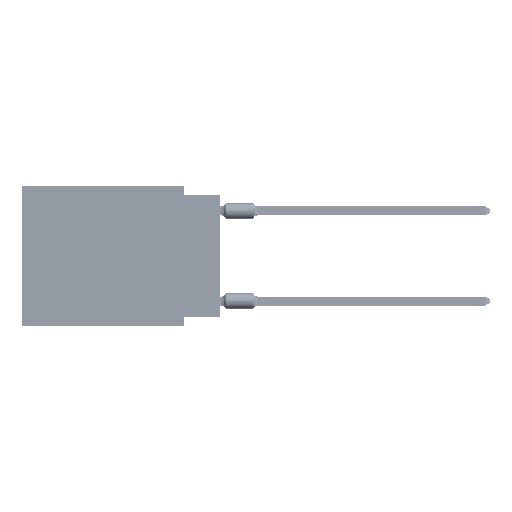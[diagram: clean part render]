
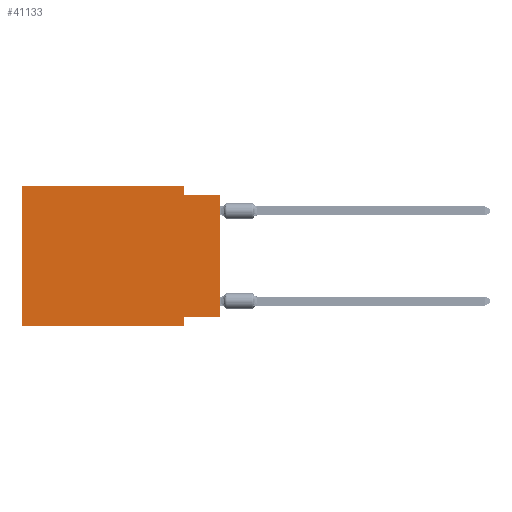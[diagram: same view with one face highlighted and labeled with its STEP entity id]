
A CAD part, left-side view. The second image highlights one B-rep face of the part: STEP entity #41133.
In plain terms, the highlighted planar face has unit normal (-1, 0, 0).
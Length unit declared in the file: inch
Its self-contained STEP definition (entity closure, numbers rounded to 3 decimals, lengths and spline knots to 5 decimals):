
#1566 = CARTESIAN_POINT ( 'NONE',  ( 0., 0., -0.025 ) ) ;
#3106 = LINE ( 'NONE', #46605, #52189 ) ;
#8135 = LINE ( 'NONE', #40934, #17220 ) ;
#8172 = EDGE_CURVE ( 'NONE', #58914, #65936, #8135, .T. ) ;
#9421 = VECTOR ( 'NONE', #50061, 39.37008 ) ;
#10401 = CARTESIAN_POINT ( 'NONE',  ( 0., 0.55, -0.39 ) ) ;
#13799 = DIRECTION ( 'NONE',  ( 0., 0., 1. ) ) ;
#14535 = CARTESIAN_POINT ( 'NONE',  ( 0., 0., -0.365 ) ) ;
#14879 = EDGE_CURVE ( 'NONE', #18918, #38628, #37913, .T. ) ;
#16019 = EDGE_CURVE ( 'NONE', #68452, #18918, #46239, .T. ) ;
#16567 = LINE ( 'NONE', #22951, #9421 ) ;
#16810 = VECTOR ( 'NONE', #13799, 39.37008 ) ;
#16828 = LINE ( 'NONE', #10401, #68112 ) ;
#17159 = DIRECTION ( 'NONE',  ( 0., -1., 0. ) ) ;
#17220 = VECTOR ( 'NONE', #62311, 39.37008 ) ;
#18135 = DIRECTION ( 'NONE',  ( 0., 0., -1. ) ) ;
#18264 = ORIENTED_EDGE ( 'NONE', *, *, #30459, .T. ) ;
#18918 = VERTEX_POINT ( 'NONE', #27631 ) ;
#18987 = FACE_OUTER_BOUND ( 'NONE', #70280, .T. ) ;
#21227 = VECTOR ( 'NONE', #37195, 39.37008 ) ;
#22951 = CARTESIAN_POINT ( 'NONE',  ( 0., 0., -0.025 ) ) ;
#23800 = ORIENTED_EDGE ( 'NONE', *, *, #62134, .T. ) ;
#23830 = LINE ( 'NONE', #61618, #54489 ) ;
#24163 = ORIENTED_EDGE ( 'NONE', *, *, #16019, .F. ) ;
#26587 = EDGE_CURVE ( 'NONE', #38628, #33888, #23830, .T. ) ;
#27631 = CARTESIAN_POINT ( 'NONE',  ( 0., 0.55, 0. ) ) ;
#29457 = CARTESIAN_POINT ( 'NONE',  ( 0., 0.1, 0. ) ) ;
#30459 = EDGE_CURVE ( 'NONE', #58914, #63016, #69448, .T. ) ;
#33888 = VERTEX_POINT ( 'NONE', #38398 ) ;
#35043 = CARTESIAN_POINT ( 'NONE',  ( 0., 0.55, 0. ) ) ;
#35385 = DIRECTION ( 'NONE',  ( 0., 0., -1. ) ) ;
#37195 = DIRECTION ( 'NONE',  ( 0., -1., 0. ) ) ;
#37747 = CARTESIAN_POINT ( 'NONE',  ( 0., 0., 0. ) ) ;
#37913 = LINE ( 'NONE', #64629, #21227 ) ;
#38398 = CARTESIAN_POINT ( 'NONE',  ( 0., 0.1, -0.025 ) ) ;
#38628 = VERTEX_POINT ( 'NONE', #29457 ) ;
#40934 = CARTESIAN_POINT ( 'NONE',  ( 0., 0., -0.365 ) ) ;
#41133 = ADVANCED_FACE ( 'NONE', ( #18987 ), #55735, .F. ) ;
#42041 = DIRECTION ( 'NONE',  ( 0., 0., 1. ) ) ;
#46239 = LINE ( 'NONE', #51564, #16810 ) ;
#46605 = CARTESIAN_POINT ( 'NONE',  ( 0., 0.1, -0.39 ) ) ;
#46675 = VERTEX_POINT ( 'NONE', #67539 ) ;
#47008 = EDGE_CURVE ( 'NONE', #33888, #63016, #16567, .T. ) ;
#47182 = ORIENTED_EDGE ( 'NONE', *, *, #57730, .F. ) ;
#47840 = ORIENTED_EDGE ( 'NONE', *, *, #47008, .F. ) ;
#48963 = CARTESIAN_POINT ( 'NONE',  ( 0., 0.1, -0.365 ) ) ;
#50061 = DIRECTION ( 'NONE',  ( 0., -1., 0. ) ) ;
#51564 = CARTESIAN_POINT ( 'NONE',  ( 0., 0.55, 0. ) ) ;
#52189 = VECTOR ( 'NONE', #57654, 39.37008 ) ;
#54489 = VECTOR ( 'NONE', #18135, 39.37008 ) ;
#55735 = PLANE ( 'NONE',  #68884 ) ;
#56776 = DIRECTION ( 'NONE',  ( 1., 0., 0. ) ) ;
#56941 = ORIENTED_EDGE ( 'NONE', *, *, #8172, .F. ) ;
#57654 = DIRECTION ( 'NONE',  ( 0., 0., -1. ) ) ;
#57730 = EDGE_CURVE ( 'NONE', #65936, #46675, #3106, .T. ) ;
#58914 = VERTEX_POINT ( 'NONE', #14535 ) ;
#60424 = VECTOR ( 'NONE', #42041, 39.37008 ) ;
#61618 = CARTESIAN_POINT ( 'NONE',  ( 0., 0.1, 0. ) ) ;
#62134 = EDGE_CURVE ( 'NONE', #68452, #46675, #16828, .T. ) ;
#62311 = DIRECTION ( 'NONE',  ( 0., 1., 0. ) ) ;
#63016 = VERTEX_POINT ( 'NONE', #1566 ) ;
#63173 = CARTESIAN_POINT ( 'NONE',  ( 0., 0.55, -0.39 ) ) ;
#63282 = ORIENTED_EDGE ( 'NONE', *, *, #14879, .F. ) ;
#64629 = CARTESIAN_POINT ( 'NONE',  ( 0., 0.55, 0. ) ) ;
#65936 = VERTEX_POINT ( 'NONE', #48963 ) ;
#67539 = CARTESIAN_POINT ( 'NONE',  ( 0., 0.1, -0.39 ) ) ;
#68112 = VECTOR ( 'NONE', #17159, 39.37008 ) ;
#68452 = VERTEX_POINT ( 'NONE', #63173 ) ;
#68884 = AXIS2_PLACEMENT_3D ( 'NONE', #35043, #56776, #35385 ) ;
#69048 = ORIENTED_EDGE ( 'NONE', *, *, #26587, .F. ) ;
#69448 = LINE ( 'NONE', #37747, #60424 ) ;
#70280 = EDGE_LOOP ( 'NONE', ( #18264, #47840, #69048, #63282, #24163, #23800, #47182, #56941 ) ) ;
